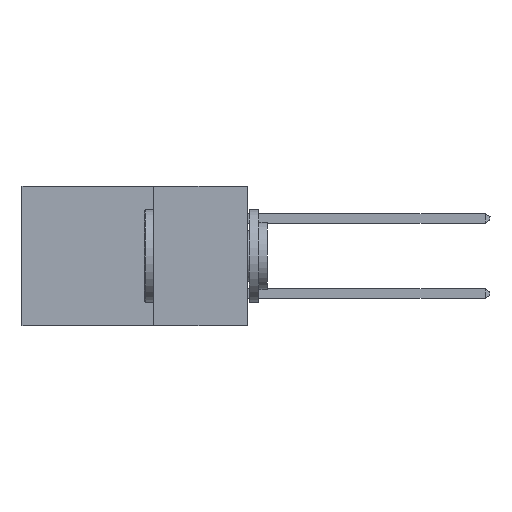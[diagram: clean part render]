
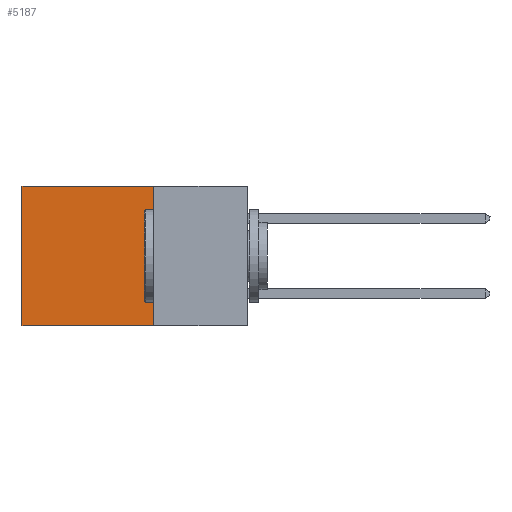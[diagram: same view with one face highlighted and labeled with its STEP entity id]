
A CAD part, left-side view. The second image highlights one B-rep face of the part: STEP entity #5187.
In plain terms, the highlighted planar face has unit normal (-1, 0, 0).
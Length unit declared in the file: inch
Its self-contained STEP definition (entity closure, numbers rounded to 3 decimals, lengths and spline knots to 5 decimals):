
#1026 = ORIENTED_EDGE ( 'NONE', *, *, #12143, .T. ) ;
#1200 = VERTEX_POINT ( 'NONE', #9259 ) ;
#1598 = VECTOR ( 'NONE', #6835, 39.37008 ) ;
#2006 = EDGE_CURVE ( 'NONE', #2304, #12018, #4881, .T. ) ;
#2023 = LINE ( 'NONE', #16788, #16158 ) ;
#2220 = DIRECTION ( 'NONE',  ( 0., 0., -1. ) ) ;
#2304 = VERTEX_POINT ( 'NONE', #16498 ) ;
#2350 = ORIENTED_EDGE ( 'NONE', *, *, #15632, .F. ) ;
#2679 = VERTEX_POINT ( 'NONE', #9730 ) ;
#3490 = FACE_OUTER_BOUND ( 'NONE', #4830, .T. ) ;
#4660 = VECTOR ( 'NONE', #10425, 39.37008 ) ;
#4830 = EDGE_LOOP ( 'NONE', ( #12285, #5242, #2350, #1026 ) ) ;
#4881 = LINE ( 'NONE', #12136, #5950 ) ;
#5187 = ADVANCED_FACE ( 'NONE', ( #3490 ), #7858, .F. ) ;
#5218 = LINE ( 'NONE', #9753, #1598 ) ;
#5242 = ORIENTED_EDGE ( 'NONE', *, *, #9853, .F. ) ;
#5463 = AXIS2_PLACEMENT_3D ( 'NONE', #16035, #17526, #2220 ) ;
#5950 = VECTOR ( 'NONE', #13397, 39.37008 ) ;
#6835 = DIRECTION ( 'NONE',  ( 0., 1., 0. ) ) ;
#7858 = PLANE ( 'NONE',  #5463 ) ;
#8922 = CARTESIAN_POINT ( 'NONE',  ( 0.298, 0.25, 0. ) ) ;
#9259 = CARTESIAN_POINT ( 'NONE',  ( 0.298, 0.25, 0. ) ) ;
#9730 = CARTESIAN_POINT ( 'NONE',  ( 0.298, 0.25, -0.37 ) ) ;
#9753 = CARTESIAN_POINT ( 'NONE',  ( 0.298, 0.25, -0.37 ) ) ;
#9853 = EDGE_CURVE ( 'NONE', #2679, #12018, #5218, .T. ) ;
#10425 = DIRECTION ( 'NONE',  ( 0., 0., -1. ) ) ;
#11404 = DIRECTION ( 'NONE',  ( 0., 1., 0. ) ) ;
#11969 = LINE ( 'NONE', #8922, #4660 ) ;
#12018 = VERTEX_POINT ( 'NONE', #14974 ) ;
#12136 = CARTESIAN_POINT ( 'NONE',  ( 0.298, 0.6, 0. ) ) ;
#12143 = EDGE_CURVE ( 'NONE', #1200, #2304, #2023, .T. ) ;
#12285 = ORIENTED_EDGE ( 'NONE', *, *, #2006, .T. ) ;
#13397 = DIRECTION ( 'NONE',  ( 0., 0., -1. ) ) ;
#14974 = CARTESIAN_POINT ( 'NONE',  ( 0.298, 0.6, -0.37 ) ) ;
#15632 = EDGE_CURVE ( 'NONE', #1200, #2679, #11969, .T. ) ;
#16035 = CARTESIAN_POINT ( 'NONE',  ( 0.298, 0.25, 0. ) ) ;
#16158 = VECTOR ( 'NONE', #11404, 39.37008 ) ;
#16498 = CARTESIAN_POINT ( 'NONE',  ( 0.298, 0.6, 0. ) ) ;
#16788 = CARTESIAN_POINT ( 'NONE',  ( 0.298, 0.25, 0. ) ) ;
#17526 = DIRECTION ( 'NONE',  ( 1., 0., 0. ) ) ;
